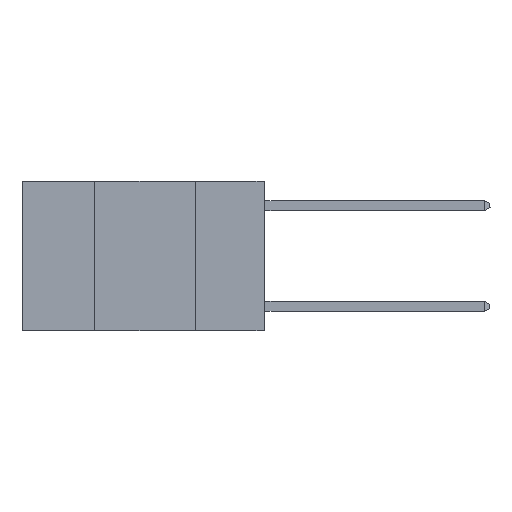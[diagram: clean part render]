
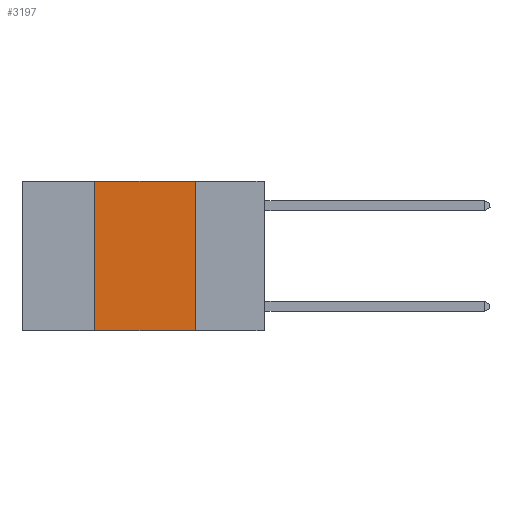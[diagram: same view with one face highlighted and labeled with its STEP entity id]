
A CAD part, left-side view. The second image highlights one B-rep face of the part: STEP entity #3197.
In plain terms, the highlighted planar face has unit normal (-1, 0, 0).
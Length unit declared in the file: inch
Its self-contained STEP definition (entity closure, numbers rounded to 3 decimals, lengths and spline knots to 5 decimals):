
#440 = DIRECTION ( 'NONE',  ( 0., -1., 0. ) ) ;
#581 = VECTOR ( 'NONE', #440, 39.37008 ) ;
#639 = ORIENTED_EDGE ( 'NONE', *, *, #9749, .F. ) ;
#884 = ORIENTED_EDGE ( 'NONE', *, *, #5119, .T. ) ;
#911 = LINE ( 'NONE', #1782, #8532 ) ;
#1077 = LINE ( 'NONE', #9798, #581 ) ;
#1141 = VECTOR ( 'NONE', #2567, 39.37008 ) ;
#1782 = CARTESIAN_POINT ( 'NONE',  ( 0., 0.42, 0. ) ) ;
#2000 = DIRECTION ( 'NONE',  ( 0., -1., 0. ) ) ;
#2567 = DIRECTION ( 'NONE',  ( 0., 0., -1. ) ) ;
#2591 = DIRECTION ( 'NONE',  ( 1., 0., 0. ) ) ;
#2637 = CARTESIAN_POINT ( 'NONE',  ( 0., 0.42, 0. ) ) ;
#3124 = CARTESIAN_POINT ( 'NONE',  ( 0., 0.17, -0.37 ) ) ;
#3197 = ADVANCED_FACE ( 'NONE', ( #4891 ), #4933, .F. ) ;
#3577 = CARTESIAN_POINT ( 'NONE',  ( 0., 0.6, 0. ) ) ;
#4321 = VERTEX_POINT ( 'NONE', #5015 ) ;
#4628 = EDGE_LOOP ( 'NONE', ( #8740, #639, #8976, #884 ) ) ;
#4891 = FACE_OUTER_BOUND ( 'NONE', #4628, .T. ) ;
#4929 = VERTEX_POINT ( 'NONE', #2637 ) ;
#4933 = PLANE ( 'NONE',  #9926 ) ;
#5015 = CARTESIAN_POINT ( 'NONE',  ( 0., 0.17, 0. ) ) ;
#5119 = EDGE_CURVE ( 'NONE', #5919, #8334, #1077, .T. ) ;
#5703 = VECTOR ( 'NONE', #2000, 39.37008 ) ;
#5735 = DIRECTION ( 'NONE',  ( 0., 0., 1. ) ) ;
#5737 = CARTESIAN_POINT ( 'NONE',  ( 0., 0.6, 0. ) ) ;
#5919 = VERTEX_POINT ( 'NONE', #8438 ) ;
#5955 = LINE ( 'NONE', #3577, #5703 ) ;
#7184 = EDGE_CURVE ( 'NONE', #5919, #4929, #911, .T. ) ;
#8095 = DIRECTION ( 'NONE',  ( 0., 0., -1. ) ) ;
#8334 = VERTEX_POINT ( 'NONE', #3124 ) ;
#8438 = CARTESIAN_POINT ( 'NONE',  ( 0., 0.42, -0.37 ) ) ;
#8494 = EDGE_CURVE ( 'NONE', #4321, #8334, #9432, .T. ) ;
#8532 = VECTOR ( 'NONE', #5735, 39.37008 ) ;
#8740 = ORIENTED_EDGE ( 'NONE', *, *, #8494, .F. ) ;
#8976 = ORIENTED_EDGE ( 'NONE', *, *, #7184, .F. ) ;
#9432 = LINE ( 'NONE', #9530, #1141 ) ;
#9530 = CARTESIAN_POINT ( 'NONE',  ( 0., 0.17, 0. ) ) ;
#9749 = EDGE_CURVE ( 'NONE', #4929, #4321, #5955, .T. ) ;
#9798 = CARTESIAN_POINT ( 'NONE',  ( 0., 0.6, -0.37 ) ) ;
#9926 = AXIS2_PLACEMENT_3D ( 'NONE', #5737, #2591, #8095 ) ;
